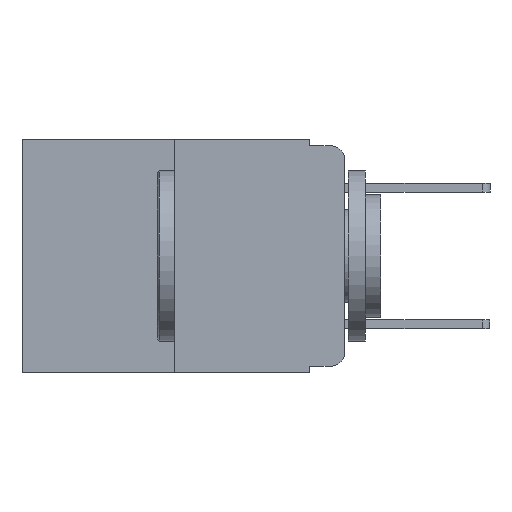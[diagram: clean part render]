
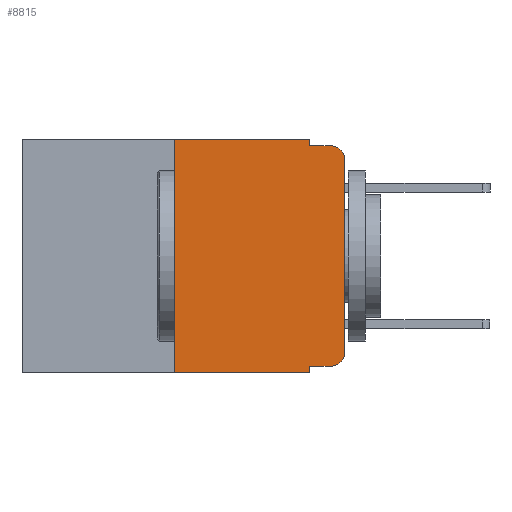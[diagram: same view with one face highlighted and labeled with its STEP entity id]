
A CAD part, left-side view. The second image highlights one B-rep face of the part: STEP entity #8815.
In plain terms, the highlighted planar face has unit normal (-1, 0, 0).
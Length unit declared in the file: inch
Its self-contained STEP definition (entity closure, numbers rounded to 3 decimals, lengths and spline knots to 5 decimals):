
#17 = ORIENTED_EDGE ( 'NONE', *, *, #7128, .T. ) ;
#62 = VECTOR ( 'NONE', #1851, 39.37008 ) ;
#166 = VERTEX_POINT ( 'NONE', #8862 ) ;
#324 = VECTOR ( 'NONE', #8394, 39.37008 ) ;
#380 = VECTOR ( 'NONE', #7229, 39.37008 ) ;
#473 = PLANE ( 'NONE',  #10867 ) ;
#553 = VERTEX_POINT ( 'NONE', #10684 ) ;
#734 = CARTESIAN_POINT ( 'NONE',  ( 0., 0., -0.03 ) ) ;
#809 = VERTEX_POINT ( 'NONE', #4151 ) ;
#1078 = LINE ( 'NONE', #1489, #2796 ) ;
#1332 = EDGE_CURVE ( 'NONE', #9187, #10034, #7303, .T. ) ;
#1428 = CARTESIAN_POINT ( 'NONE',  ( 0., 0.25, 0. ) ) ;
#1462 = DIRECTION ( 'NONE',  ( 1., 0., 0. ) ) ;
#1489 = CARTESIAN_POINT ( 'NONE',  ( 0., 0., 0. ) ) ;
#1599 = CARTESIAN_POINT ( 'NONE',  ( 0., 0.473, -0.343 ) ) ;
#1677 = VECTOR ( 'NONE', #5889, 39.37008 ) ;
#1734 = DIRECTION ( 'NONE',  ( -1., 0., 0. ) ) ;
#1779 = ORIENTED_EDGE ( 'NONE', *, *, #5191, .F. ) ;
#1785 = ORIENTED_EDGE ( 'NONE', *, *, #3497, .T. ) ;
#1851 = DIRECTION ( 'NONE',  ( 0., 0., 1. ) ) ;
#1895 = ORIENTED_EDGE ( 'NONE', *, *, #2882, .F. ) ;
#1918 = VECTOR ( 'NONE', #5051, 39.37008 ) ;
#2235 = ORIENTED_EDGE ( 'NONE', *, *, #4208, .T. ) ;
#2314 = CARTESIAN_POINT ( 'NONE',  ( 0., 0.051, 0. ) ) ;
#2490 = VERTEX_POINT ( 'NONE', #7165 ) ;
#2625 = DIRECTION ( 'NONE',  ( 0., -1., 0. ) ) ;
#2710 = ORIENTED_EDGE ( 'NONE', *, *, #4245, .T. ) ;
#2796 = VECTOR ( 'NONE', #7690, 39.37008 ) ;
#2882 = EDGE_CURVE ( 'NONE', #809, #8419, #5352, .T. ) ;
#2977 = AXIS2_PLACEMENT_3D ( 'NONE', #7020, #1734, #7842 ) ;
#3244 = CARTESIAN_POINT ( 'NONE',  ( 0., 0.02, -0.313 ) ) ;
#3497 = EDGE_CURVE ( 'NONE', #809, #2490, #4398, .T. ) ;
#3522 = EDGE_CURVE ( 'NONE', #10034, #553, #8783, .T. ) ;
#3832 = CIRCLE ( 'NONE', #2977, 0.02 ) ;
#4151 = CARTESIAN_POINT ( 'NONE',  ( 0., 0.051, -0.333 ) ) ;
#4157 = DIRECTION ( 'NONE',  ( 0., 0., -1. ) ) ;
#4208 = EDGE_CURVE ( 'NONE', #9187, #8419, #9897, .T. ) ;
#4245 = EDGE_CURVE ( 'NONE', #5385, #166, #3832, .T. ) ;
#4398 = LINE ( 'NONE', #9083, #10643 ) ;
#4881 = ORIENTED_EDGE ( 'NONE', *, *, #11024, .T. ) ;
#5009 = DIRECTION ( 'NONE',  ( 0., -1., 0. ) ) ;
#5051 = DIRECTION ( 'NONE',  ( 0., -1., 0. ) ) ;
#5191 = EDGE_CURVE ( 'NONE', #7464, #166, #7237, .T. ) ;
#5352 = LINE ( 'NONE', #6398, #380 ) ;
#5385 = VERTEX_POINT ( 'NONE', #734 ) ;
#5508 = CARTESIAN_POINT ( 'NONE',  ( 0., 0., -0.313 ) ) ;
#5554 = CARTESIAN_POINT ( 'NONE',  ( 0., 0.25, 0. ) ) ;
#5889 = DIRECTION ( 'NONE',  ( 0., 0., -1. ) ) ;
#6398 = CARTESIAN_POINT ( 'NONE',  ( 0., 0.051, 0. ) ) ;
#6538 = ORIENTED_EDGE ( 'NONE', *, *, #1332, .F. ) ;
#6633 = ORIENTED_EDGE ( 'NONE', *, *, #3522, .F. ) ;
#7020 = CARTESIAN_POINT ( 'NONE',  ( 0., 0.02, -0.03 ) ) ;
#7128 = EDGE_CURVE ( 'NONE', #2490, #8438, #9355, .T. ) ;
#7165 = CARTESIAN_POINT ( 'NONE',  ( 0., 0.02, -0.333 ) ) ;
#7229 = DIRECTION ( 'NONE',  ( 0., 0., -1. ) ) ;
#7237 = LINE ( 'NONE', #10766, #324 ) ;
#7303 = LINE ( 'NONE', #5554, #62 ) ;
#7464 = VERTEX_POINT ( 'NONE', #9460 ) ;
#7483 = FACE_OUTER_BOUND ( 'NONE', #9733, .T. ) ;
#7621 = DIRECTION ( 'NONE',  ( 0., 0., -1. ) ) ;
#7690 = DIRECTION ( 'NONE',  ( 0., 0., 1. ) ) ;
#7842 = DIRECTION ( 'NONE',  ( 0., 0., -1. ) ) ;
#8394 = DIRECTION ( 'NONE',  ( 0., -1., 0. ) ) ;
#8419 = VERTEX_POINT ( 'NONE', #11130 ) ;
#8438 = VERTEX_POINT ( 'NONE', #5508 ) ;
#8496 = ORIENTED_EDGE ( 'NONE', *, *, #10898, .F. ) ;
#8783 = LINE ( 'NONE', #9912, #1918 ) ;
#8815 = ADVANCED_FACE ( 'NONE', ( #7483 ), #473, .F. ) ;
#8845 = CARTESIAN_POINT ( 'NONE',  ( 0., 0.25, -0.343 ) ) ;
#8862 = CARTESIAN_POINT ( 'NONE',  ( 0., 0.02, -0.01 ) ) ;
#9083 = CARTESIAN_POINT ( 'NONE',  ( 0., 0.051, -0.333 ) ) ;
#9106 = DIRECTION ( 'NONE',  ( -1., 0., 0. ) ) ;
#9187 = VERTEX_POINT ( 'NONE', #8845 ) ;
#9355 = CIRCLE ( 'NONE', #10252, 0.02 ) ;
#9460 = CARTESIAN_POINT ( 'NONE',  ( 0., 0.051, -0.01 ) ) ;
#9733 = EDGE_LOOP ( 'NONE', ( #4881, #2710, #1779, #8496, #6633, #6538, #2235, #1895, #1785, #17 ) ) ;
#9897 = LINE ( 'NONE', #1599, #10149 ) ;
#9912 = CARTESIAN_POINT ( 'NONE',  ( 0., 0.473, 0. ) ) ;
#10034 = VERTEX_POINT ( 'NONE', #1428 ) ;
#10149 = VECTOR ( 'NONE', #2625, 39.37008 ) ;
#10252 = AXIS2_PLACEMENT_3D ( 'NONE', #3244, #9106, #4157 ) ;
#10643 = VECTOR ( 'NONE', #5009, 39.37008 ) ;
#10684 = CARTESIAN_POINT ( 'NONE',  ( 0., 0.051, 0. ) ) ;
#10764 = CARTESIAN_POINT ( 'NONE',  ( 0., 0.473, 0. ) ) ;
#10766 = CARTESIAN_POINT ( 'NONE',  ( 0., 0.051, -0.01 ) ) ;
#10867 = AXIS2_PLACEMENT_3D ( 'NONE', #10764, #1462, #7621 ) ;
#10898 = EDGE_CURVE ( 'NONE', #553, #7464, #10968, .T. ) ;
#10968 = LINE ( 'NONE', #2314, #1677 ) ;
#11024 = EDGE_CURVE ( 'NONE', #8438, #5385, #1078, .T. ) ;
#11130 = CARTESIAN_POINT ( 'NONE',  ( 0., 0.051, -0.343 ) ) ;
